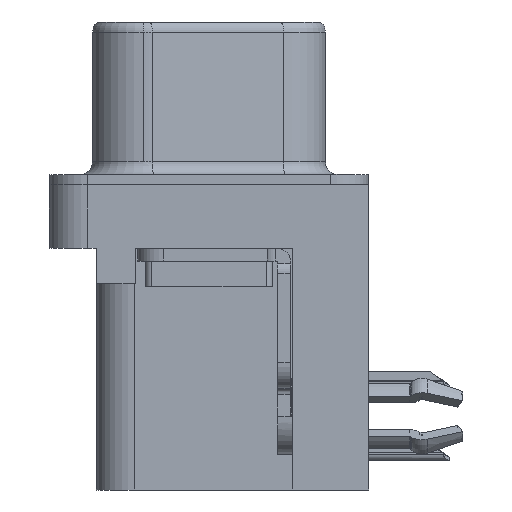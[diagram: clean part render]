
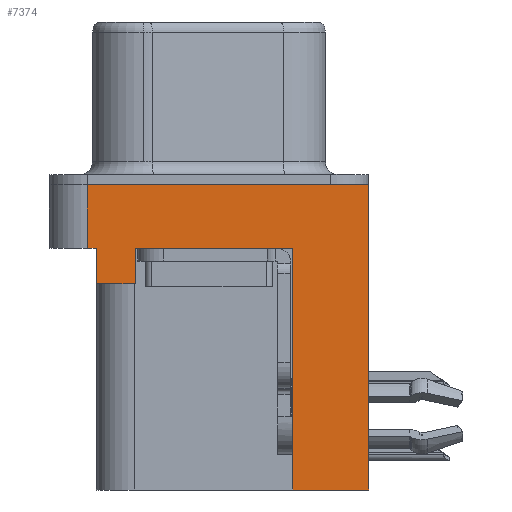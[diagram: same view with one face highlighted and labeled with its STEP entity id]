
A CAD part, left-side view. The second image highlights one B-rep face of the part: STEP entity #7374.
In plain terms, the highlighted planar face has unit normal (-1, 0, 0).
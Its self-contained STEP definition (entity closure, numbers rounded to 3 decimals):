
#367 = ORIENTED_EDGE ( 'NONE', *, *, #28456, .T. ) ;
#524 = CARTESIAN_POINT ( 'NONE',  ( -2.91, -6.275, -2.5 ) ) ;
#1734 = EDGE_CURVE ( 'NONE', #16567, #11093, #25006, .T. ) ;
#1750 = VECTOR ( 'NONE', #3206, 1000. ) ;
#1976 = CARTESIAN_POINT ( 'NONE',  ( -2.91, -6.275, 0. ) ) ;
#2893 = VERTEX_POINT ( 'NONE', #7613 ) ;
#3206 = DIRECTION ( 'NONE',  ( 0., -1., 0. ) ) ;
#3209 = DIRECTION ( 'NONE',  ( 0., 0., 1. ) ) ;
#4162 = LINE ( 'NONE', #25203, #21466 ) ;
#4532 = VECTOR ( 'NONE', #5856, 1000. ) ;
#4677 = EDGE_CURVE ( 'NONE', #11093, #14411, #13107, .T. ) ;
#4762 = DIRECTION ( 'NONE',  ( 0., 0., 1. ) ) ;
#4819 = EDGE_CURVE ( 'NONE', #8396, #7307, #28121, .T. ) ;
#5825 = ORIENTED_EDGE ( 'NONE', *, *, #14987, .T. ) ;
#5856 = DIRECTION ( 'NONE',  ( 0., 0., 1. ) ) ;
#6259 = CARTESIAN_POINT ( 'NONE',  ( -2.91, 4.425, -2.5 ) ) ;
#6435 = VERTEX_POINT ( 'NONE', #6259 ) ;
#7051 = ORIENTED_EDGE ( 'NONE', *, *, #28026, .F. ) ;
#7307 = VERTEX_POINT ( 'NONE', #8786 ) ;
#7374 = ADVANCED_FACE ( 'NONE', ( #15241 ), #24076, .T. ) ;
#7613 = CARTESIAN_POINT ( 'NONE',  ( -2.91, -3.295, -2.5 ) ) ;
#7854 = VERTEX_POINT ( 'NONE', #8445 ) ;
#8396 = VERTEX_POINT ( 'NONE', #12121 ) ;
#8445 = CARTESIAN_POINT ( 'NONE',  ( -2.91, 4.425, -3.9 ) ) ;
#8540 = LINE ( 'NONE', #9162, #22388 ) ;
#8786 = CARTESIAN_POINT ( 'NONE',  ( -2.91, 2.895, -2.5 ) ) ;
#9162 = CARTESIAN_POINT ( 'NONE',  ( -2.91, 4.425, -3.9 ) ) ;
#9243 = DIRECTION ( 'NONE',  ( 0., 1., 0. ) ) ;
#9623 = VECTOR ( 'NONE', #4762, 1000. ) ;
#10151 = CARTESIAN_POINT ( 'NONE',  ( -2.91, 4.775, -2.5 ) ) ;
#10380 = CARTESIAN_POINT ( 'NONE',  ( -2.91, 4.425, -3.9 ) ) ;
#10388 = DIRECTION ( 'NONE',  ( 0., -1., 0. ) ) ;
#11047 = ORIENTED_EDGE ( 'NONE', *, *, #1734, .F. ) ;
#11093 = VERTEX_POINT ( 'NONE', #25028 ) ;
#11287 = CARTESIAN_POINT ( 'NONE',  ( -2.91, -6.275, -12. ) ) ;
#11565 = DIRECTION ( 'NONE',  ( 0., -1., 0. ) ) ;
#11585 = AXIS2_PLACEMENT_3D ( 'NONE', #24366, #21932, #22105 ) ;
#11987 = CARTESIAN_POINT ( 'NONE',  ( -2.91, 4.775, -2.5 ) ) ;
#12121 = CARTESIAN_POINT ( 'NONE',  ( -2.91, 2.895, -3.9 ) ) ;
#12590 = CARTESIAN_POINT ( 'NONE',  ( -2.91, -3.295, -12. ) ) ;
#12769 = CARTESIAN_POINT ( 'NONE',  ( -2.91, -3.295, -12. ) ) ;
#13107 = LINE ( 'NONE', #17070, #14137 ) ;
#14137 = VECTOR ( 'NONE', #10388, 1000. ) ;
#14213 = EDGE_CURVE ( 'NONE', #7854, #6435, #19916, .T. ) ;
#14411 = VERTEX_POINT ( 'NONE', #1976 ) ;
#14667 = ORIENTED_EDGE ( 'NONE', *, *, #20133, .T. ) ;
#14742 = VERTEX_POINT ( 'NONE', #15071 ) ;
#14940 = VERTEX_POINT ( 'NONE', #11287 ) ;
#14987 = EDGE_CURVE ( 'NONE', #14940, #14411, #15535, .T. ) ;
#15071 = CARTESIAN_POINT ( 'NONE',  ( -2.91, -3.295, -12. ) ) ;
#15241 = FACE_OUTER_BOUND ( 'NONE', #28078, .T. ) ;
#15535 = LINE ( 'NONE', #524, #9623 ) ;
#16273 = LINE ( 'NONE', #12590, #4532 ) ;
#16567 = VERTEX_POINT ( 'NONE', #11987 ) ;
#17070 = CARTESIAN_POINT ( 'NONE',  ( -2.91, -6.275, 0. ) ) ;
#18979 = CARTESIAN_POINT ( 'NONE',  ( -2.91, -6.275, -2.5 ) ) ;
#19579 = DIRECTION ( 'NONE',  ( 0., 1., 0. ) ) ;
#19916 = LINE ( 'NONE', #10380, #27487 ) ;
#20047 = ORIENTED_EDGE ( 'NONE', *, *, #4819, .T. ) ;
#20133 = EDGE_CURVE ( 'NONE', #7307, #2893, #24879, .T. ) ;
#21439 = ORIENTED_EDGE ( 'NONE', *, *, #25881, .F. ) ;
#21466 = VECTOR ( 'NONE', #11565, 1000. ) ;
#21668 = ORIENTED_EDGE ( 'NONE', *, *, #4677, .F. ) ;
#21914 = VECTOR ( 'NONE', #3209, 1000. ) ;
#21932 = DIRECTION ( 'NONE',  ( -1., 0., 0. ) ) ;
#22105 = DIRECTION ( 'NONE',  ( 0., 0., 1. ) ) ;
#22388 = VECTOR ( 'NONE', #9243, 1000. ) ;
#23323 = VECTOR ( 'NONE', #26471, 1000. ) ;
#23868 = ORIENTED_EDGE ( 'NONE', *, *, #24368, .F. ) ;
#24076 = PLANE ( 'NONE',  #11585 ) ;
#24366 = CARTESIAN_POINT ( 'NONE',  ( -2.91, -6.275, -2.5 ) ) ;
#24368 = EDGE_CURVE ( 'NONE', #14940, #14742, #24605, .T. ) ;
#24605 = LINE ( 'NONE', #12769, #28361 ) ;
#24879 = LINE ( 'NONE', #18979, #1750 ) ;
#25006 = LINE ( 'NONE', #10151, #21914 ) ;
#25028 = CARTESIAN_POINT ( 'NONE',  ( -2.91, 4.775, 0. ) ) ;
#25203 = CARTESIAN_POINT ( 'NONE',  ( -2.91, -6.275, -2.5 ) ) ;
#25881 = EDGE_CURVE ( 'NONE', #8396, #7854, #8540, .T. ) ;
#26176 = CARTESIAN_POINT ( 'NONE',  ( -2.91, 2.895, -3.9 ) ) ;
#26471 = DIRECTION ( 'NONE',  ( 0., 0., 1. ) ) ;
#27487 = VECTOR ( 'NONE', #28048, 1000. ) ;
#28026 = EDGE_CURVE ( 'NONE', #14742, #2893, #16273, .T. ) ;
#28048 = DIRECTION ( 'NONE',  ( 0., 0., 1. ) ) ;
#28078 = EDGE_LOOP ( 'NONE', ( #21668, #11047, #367, #28308, #21439, #20047, #14667, #7051, #23868, #5825 ) ) ;
#28121 = LINE ( 'NONE', #26176, #23323 ) ;
#28308 = ORIENTED_EDGE ( 'NONE', *, *, #14213, .F. ) ;
#28361 = VECTOR ( 'NONE', #19579, 1000. ) ;
#28456 = EDGE_CURVE ( 'NONE', #16567, #6435, #4162, .T. ) ;
